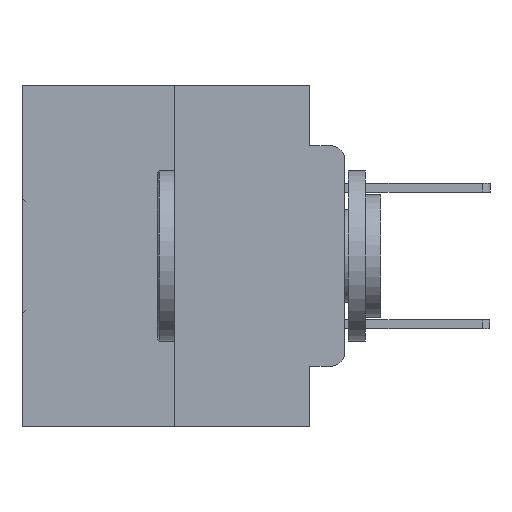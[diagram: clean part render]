
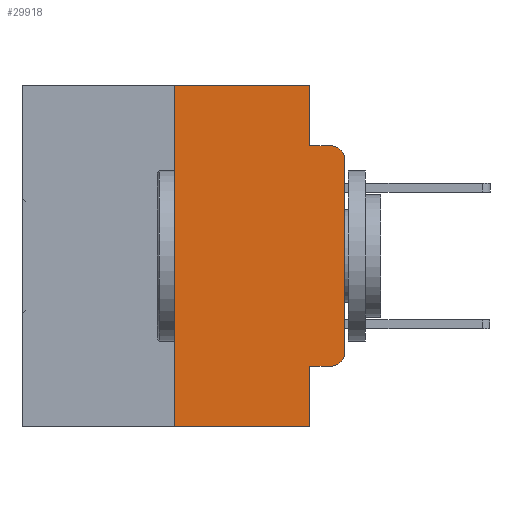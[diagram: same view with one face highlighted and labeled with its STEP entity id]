
A CAD part, left-side view. The second image highlights one B-rep face of the part: STEP entity #29918.
In plain terms, the highlighted planar face has unit normal (-1, 0, 0).
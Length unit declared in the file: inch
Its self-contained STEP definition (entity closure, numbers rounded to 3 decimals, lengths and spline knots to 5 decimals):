
#130 = CIRCLE ( 'NONE', #23196, 0.02 ) ;
#152 = CIRCLE ( 'NONE', #30536, 0.02 ) ;
#696 = EDGE_CURVE ( 'NONE', #13380, #1296, #2650, .T. ) ;
#1296 = VERTEX_POINT ( 'NONE', #7346 ) ;
#1328 = ORIENTED_EDGE ( 'NONE', *, *, #23635, .F. ) ;
#1424 = AXIS2_PLACEMENT_3D ( 'NONE', #15525, #5876, #18059 ) ;
#1877 = VECTOR ( 'NONE', #31232, 39.37008 ) ;
#2650 = LINE ( 'NONE', #31397, #28872 ) ;
#2749 = DIRECTION ( 'NONE',  ( 0., 0., 1. ) ) ;
#3023 = DIRECTION ( 'NONE',  ( -1., 0., 0. ) ) ;
#3613 = ORIENTED_EDGE ( 'NONE', *, *, #21972, .T. ) ;
#3783 = DIRECTION ( 'NONE',  ( 0., 0., -1. ) ) ;
#4532 = VERTEX_POINT ( 'NONE', #25491 ) ;
#5255 = CARTESIAN_POINT ( 'NONE',  ( 0., 0.25, 0. ) ) ;
#5876 = DIRECTION ( 'NONE',  ( 1., 0., 0. ) ) ;
#5934 = VERTEX_POINT ( 'NONE', #19060 ) ;
#6174 = LINE ( 'NONE', #26549, #26362 ) ;
#6276 = CARTESIAN_POINT ( 'NONE',  ( 0., 0.02, -0.1085 ) ) ;
#7125 = LINE ( 'NONE', #24747, #12349 ) ;
#7346 = CARTESIAN_POINT ( 'NONE',  ( 0., 0.02, -0.0885 ) ) ;
#7759 = EDGE_CURVE ( 'NONE', #9833, #1296, #130, .T. ) ;
#8901 = DIRECTION ( 'NONE',  ( 0., 0., -1. ) ) ;
#9232 = CARTESIAN_POINT ( 'NONE',  ( 0., 0., -0.1085 ) ) ;
#9514 = EDGE_CURVE ( 'NONE', #31789, #9833, #31144, .T. ) ;
#9658 = LINE ( 'NONE', #26302, #1877 ) ;
#9833 = VERTEX_POINT ( 'NONE', #9232 ) ;
#11090 = VECTOR ( 'NONE', #2749, 39.37008 ) ;
#11932 = CARTESIAN_POINT ( 'NONE',  ( 0., 0., -0.3915 ) ) ;
#11966 = CARTESIAN_POINT ( 'NONE',  ( 0., 0.473, -0.5 ) ) ;
#12096 = VERTEX_POINT ( 'NONE', #19600 ) ;
#12318 = DIRECTION ( 'NONE',  ( 0., 0., 1. ) ) ;
#12349 = VECTOR ( 'NONE', #27267, 39.37008 ) ;
#13130 = LINE ( 'NONE', #11966, #25718 ) ;
#13380 = VERTEX_POINT ( 'NONE', #14790 ) ;
#13789 = EDGE_CURVE ( 'NONE', #25837, #12096, #9658, .T. ) ;
#13975 = LINE ( 'NONE', #24827, #25748 ) ;
#14790 = CARTESIAN_POINT ( 'NONE',  ( 0., 0.051, -0.0885 ) ) ;
#15407 = VECTOR ( 'NONE', #20496, 39.37008 ) ;
#15427 = CARTESIAN_POINT ( 'NONE',  ( 0., 0.051, 0. ) ) ;
#15525 = CARTESIAN_POINT ( 'NONE',  ( 0., 0.473, 0. ) ) ;
#16022 = VERTEX_POINT ( 'NONE', #20043 ) ;
#16908 = EDGE_CURVE ( 'NONE', #4532, #31789, #152, .T. ) ;
#17111 = ORIENTED_EDGE ( 'NONE', *, *, #7759, .T. ) ;
#17738 = ORIENTED_EDGE ( 'NONE', *, *, #9514, .T. ) ;
#18059 = DIRECTION ( 'NONE',  ( 0., 0., -1. ) ) ;
#18345 = CARTESIAN_POINT ( 'NONE',  ( 0., 0.02, -0.3915 ) ) ;
#19060 = CARTESIAN_POINT ( 'NONE',  ( 0., 0.051, -0.5 ) ) ;
#19338 = ORIENTED_EDGE ( 'NONE', *, *, #32058, .F. ) ;
#19600 = CARTESIAN_POINT ( 'NONE',  ( 0., 0.051, 0. ) ) ;
#20043 = CARTESIAN_POINT ( 'NONE',  ( 0., 0.051, -0.4115 ) ) ;
#20496 = DIRECTION ( 'NONE',  ( 0., 0., -1. ) ) ;
#20628 = CARTESIAN_POINT ( 'NONE',  ( 0., 0., 0. ) ) ;
#20887 = DIRECTION ( 'NONE',  ( 0., 0., -1. ) ) ;
#21972 = EDGE_CURVE ( 'NONE', #16022, #4532, #7125, .T. ) ;
#22871 = LINE ( 'NONE', #15427, #15407 ) ;
#23196 = AXIS2_PLACEMENT_3D ( 'NONE', #6276, #24000, #8901 ) ;
#23635 = EDGE_CURVE ( 'NONE', #16022, #5934, #6174, .T. ) ;
#24000 = DIRECTION ( 'NONE',  ( -1., 0., 0. ) ) ;
#24292 = VERTEX_POINT ( 'NONE', #31563 ) ;
#24747 = CARTESIAN_POINT ( 'NONE',  ( 0., 0.051, -0.4115 ) ) ;
#24749 = EDGE_LOOP ( 'NONE', ( #17738, #17111, #25217, #19338, #32716, #28117, #29258, #1328, #3613, #29222 ) ) ;
#24827 = CARTESIAN_POINT ( 'NONE',  ( 0., 0.25, 0. ) ) ;
#25217 = ORIENTED_EDGE ( 'NONE', *, *, #696, .F. ) ;
#25491 = CARTESIAN_POINT ( 'NONE',  ( 0., 0.02, -0.4115 ) ) ;
#25718 = VECTOR ( 'NONE', #29532, 39.37008 ) ;
#25748 = VECTOR ( 'NONE', #12318, 39.37008 ) ;
#25837 = VERTEX_POINT ( 'NONE', #5255 ) ;
#26302 = CARTESIAN_POINT ( 'NONE',  ( 0., 0.473, 0. ) ) ;
#26362 = VECTOR ( 'NONE', #3783, 39.37008 ) ;
#26549 = CARTESIAN_POINT ( 'NONE',  ( 0., 0.051, 0. ) ) ;
#27267 = DIRECTION ( 'NONE',  ( 0., -1., 0. ) ) ;
#27348 = FACE_OUTER_BOUND ( 'NONE', #24749, .T. ) ;
#28117 = ORIENTED_EDGE ( 'NONE', *, *, #30336, .F. ) ;
#28872 = VECTOR ( 'NONE', #31471, 39.37008 ) ;
#29222 = ORIENTED_EDGE ( 'NONE', *, *, #16908, .T. ) ;
#29258 = ORIENTED_EDGE ( 'NONE', *, *, #30779, .T. ) ;
#29532 = DIRECTION ( 'NONE',  ( 0., -1., 0. ) ) ;
#29918 = ADVANCED_FACE ( 'NONE', ( #27348 ), #30544, .F. ) ;
#30336 = EDGE_CURVE ( 'NONE', #24292, #25837, #13975, .T. ) ;
#30536 = AXIS2_PLACEMENT_3D ( 'NONE', #18345, #3023, #20887 ) ;
#30544 = PLANE ( 'NONE',  #1424 ) ;
#30779 = EDGE_CURVE ( 'NONE', #24292, #5934, #13130, .T. ) ;
#31144 = LINE ( 'NONE', #20628, #11090 ) ;
#31232 = DIRECTION ( 'NONE',  ( 0., -1., 0. ) ) ;
#31397 = CARTESIAN_POINT ( 'NONE',  ( 0., 0.051, -0.0885 ) ) ;
#31471 = DIRECTION ( 'NONE',  ( 0., -1., 0. ) ) ;
#31563 = CARTESIAN_POINT ( 'NONE',  ( 0., 0.25, -0.5 ) ) ;
#31789 = VERTEX_POINT ( 'NONE', #11932 ) ;
#32058 = EDGE_CURVE ( 'NONE', #12096, #13380, #22871, .T. ) ;
#32716 = ORIENTED_EDGE ( 'NONE', *, *, #13789, .F. ) ;
